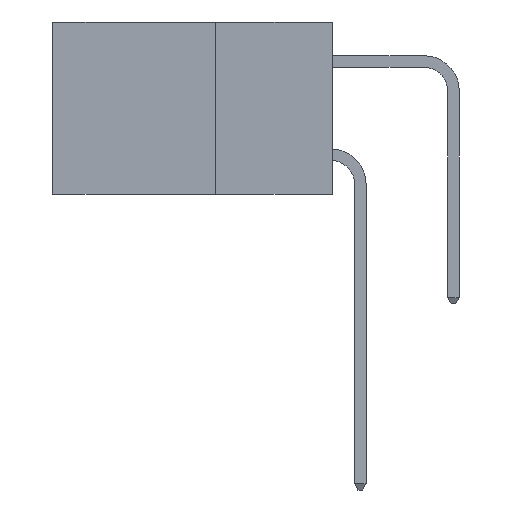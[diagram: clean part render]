
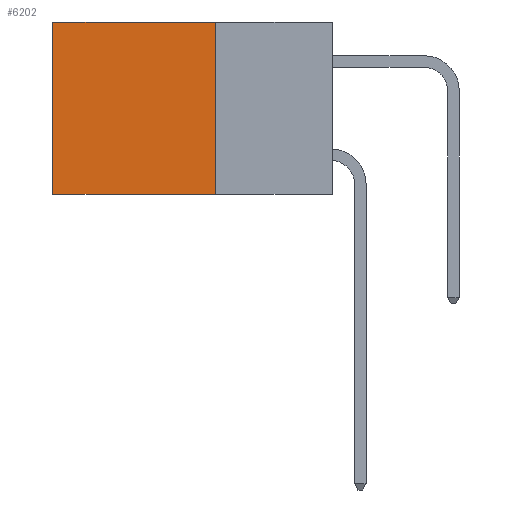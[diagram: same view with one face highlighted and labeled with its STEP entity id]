
A CAD part, left-side view. The second image highlights one B-rep face of the part: STEP entity #6202.
In plain terms, the highlighted planar face has unit normal (-1, 0, 0).
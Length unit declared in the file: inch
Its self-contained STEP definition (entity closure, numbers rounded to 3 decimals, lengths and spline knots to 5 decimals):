
#10 = PLANE ( 'NONE',  #19873 ) ;
#412 = DIRECTION ( 'NONE',  ( 1., 0., 0. ) ) ;
#723 = DIRECTION ( 'NONE',  ( 0., 0., -1. ) ) ;
#1064 = VERTEX_POINT ( 'NONE', #4112 ) ;
#1290 = VERTEX_POINT ( 'NONE', #11846 ) ;
#1920 = EDGE_CURVE ( 'NONE', #15347, #8220, #3970, .T. ) ;
#2000 = CARTESIAN_POINT ( 'NONE',  ( 0.2615, 0.25, -0.37 ) ) ;
#2041 = LINE ( 'NONE', #7259, #6424 ) ;
#2278 = CARTESIAN_POINT ( 'NONE',  ( 0.2615, 0.25, -0.37 ) ) ;
#3583 = DIRECTION ( 'NONE',  ( 0., 1., 0. ) ) ;
#3635 = EDGE_CURVE ( 'NONE', #15347, #1064, #22495, .T. ) ;
#3970 = LINE ( 'NONE', #2278, #12973 ) ;
#4112 = CARTESIAN_POINT ( 'NONE',  ( 0.2615, 0.6, 0. ) ) ;
#6202 = ADVANCED_FACE ( 'NONE', ( #10025 ), #10, .F. ) ;
#6329 = VECTOR ( 'NONE', #723, 39.37008 ) ;
#6424 = VECTOR ( 'NONE', #3583, 39.37008 ) ;
#7259 = CARTESIAN_POINT ( 'NONE',  ( 0.2615, 0.25, -0.37 ) ) ;
#7303 = ORIENTED_EDGE ( 'NONE', *, *, #3635, .T. ) ;
#7731 = EDGE_CURVE ( 'NONE', #1064, #1290, #11623, .T. ) ;
#8220 = VERTEX_POINT ( 'NONE', #21771 ) ;
#10025 = FACE_OUTER_BOUND ( 'NONE', #17207, .T. ) ;
#11623 = LINE ( 'NONE', #16936, #6329 ) ;
#11846 = CARTESIAN_POINT ( 'NONE',  ( 0.2615, 0.6, -0.37 ) ) ;
#12973 = VECTOR ( 'NONE', #16243, 39.37008 ) ;
#15237 = CARTESIAN_POINT ( 'NONE',  ( 0.2615, 0.25, 0. ) ) ;
#15347 = VERTEX_POINT ( 'NONE', #15237 ) ;
#15699 = EDGE_CURVE ( 'NONE', #8220, #1290, #2041, .T. ) ;
#16243 = DIRECTION ( 'NONE',  ( 0., 0., -1. ) ) ;
#16936 = CARTESIAN_POINT ( 'NONE',  ( 0.2615, 0.6, -0.37 ) ) ;
#17207 = EDGE_LOOP ( 'NONE', ( #22372, #22079, #22519, #7303 ) ) ;
#17267 = VECTOR ( 'NONE', #18106, 39.37008 ) ;
#18106 = DIRECTION ( 'NONE',  ( 0., 1., 0. ) ) ;
#18740 = CARTESIAN_POINT ( 'NONE',  ( 0.2615, 0.25, 0. ) ) ;
#19873 = AXIS2_PLACEMENT_3D ( 'NONE', #2000, #412, #22974 ) ;
#21771 = CARTESIAN_POINT ( 'NONE',  ( 0.2615, 0.25, -0.37 ) ) ;
#22079 = ORIENTED_EDGE ( 'NONE', *, *, #15699, .F. ) ;
#22372 = ORIENTED_EDGE ( 'NONE', *, *, #7731, .T. ) ;
#22495 = LINE ( 'NONE', #18740, #17267 ) ;
#22519 = ORIENTED_EDGE ( 'NONE', *, *, #1920, .F. ) ;
#22974 = DIRECTION ( 'NONE',  ( 0., 0., -1. ) ) ;
